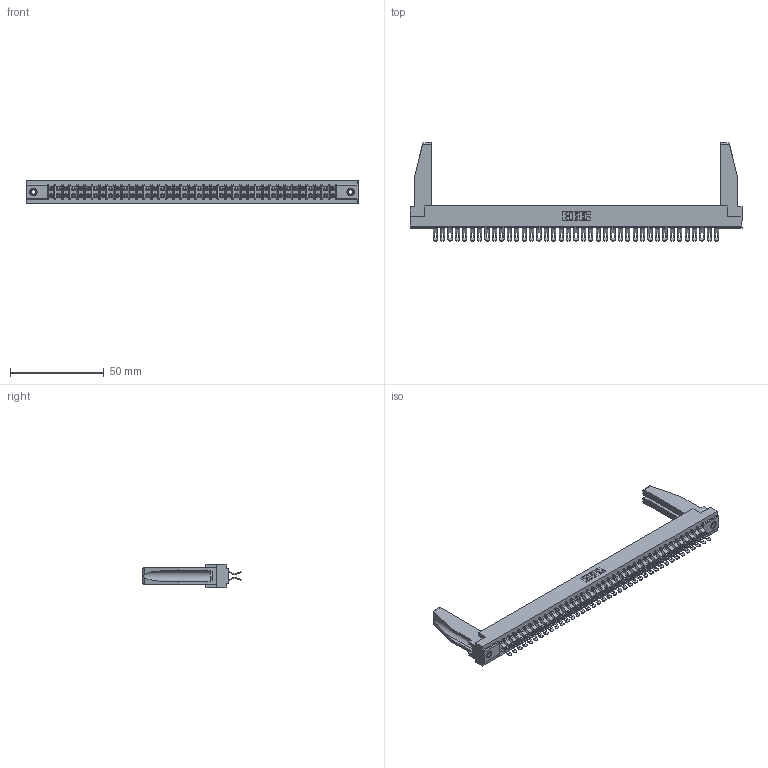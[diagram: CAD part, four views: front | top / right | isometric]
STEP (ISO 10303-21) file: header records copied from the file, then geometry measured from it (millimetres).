
FILE_DESCRIPTION (( 'STEP AP203' ), '1' );
FILE_NAME ('307-078-455-278.STEP', '2020-10-01T07:15:11', ( '' ), ( '' ), 'SwSTEP 2.0', 'SolidWorks 2020', '' );
FILE_SCHEMA (( 'CONFIG_CONTROL_DESIGN' ));
Length unit declared in the file: inch
Products named in the file (5): 307-290-001_555; 307-078-455-278; 345-250-001_345-250-001-102; 307 Part_.156 Dia Mounting Holes; 307-220-078
Assembly tree (83 placements, depth 2):
  307-078-455-278
    307 Part_.156 Dia Mounting Holes
    307-290-001_555  x78
    307-220-078  x2
    345-250-001_345-250-001-102  x2
Bounding box: 177.55 x 52.45 x 12.7 mm (x, y, z)
Volume: 23084.4 mm3; surface area: 28414.8 mm2
Topology: 83 solids, 83 shells, 5046 faces, 14771 edges, 9626 vertices
Faces by surface type: plane 2806, cylinder 2144, sphere 80, cone 12, torus 4
Entity records: 38028 total; most frequent: CARTESIAN_POINT 6237, ORIENTED_EDGE 6142, DIRECTION 6071, EDGE_CURVE 3071, LINE 2347, VECTOR 2347, VERTEX_POINT 1986, AXIS2_PLACEMENT_3D 1862
